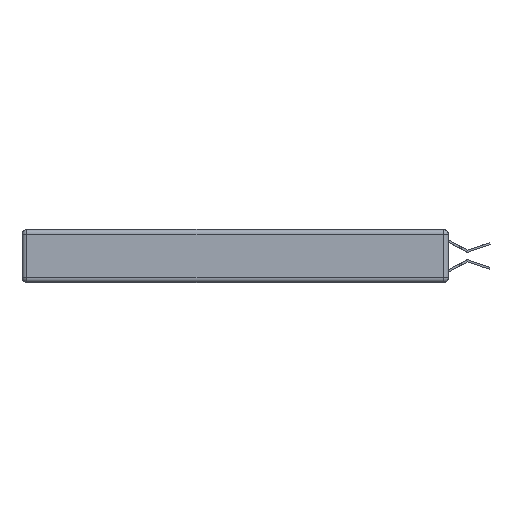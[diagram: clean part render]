
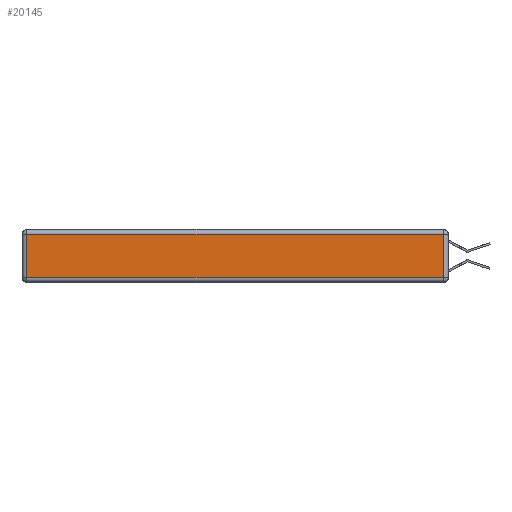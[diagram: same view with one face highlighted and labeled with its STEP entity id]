
A CAD part, left-side view. The second image highlights one B-rep face of the part: STEP entity #20145.
In plain terms, the highlighted planar face has unit normal (-1, 0, 0).
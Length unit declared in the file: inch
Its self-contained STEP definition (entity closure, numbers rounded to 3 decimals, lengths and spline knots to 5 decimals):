
#944 = DIRECTION ( 'NONE',  ( 0., 0., 1. ) ) ;
#1008 = ORIENTED_EDGE ( 'NONE', *, *, #22902, .T. ) ;
#3043 = CARTESIAN_POINT ( 'NONE',  ( 0., 0.03, -0.343 ) ) ;
#3604 = EDGE_LOOP ( 'NONE', ( #24940, #20591, #23111, #1008 ) ) ;
#4752 = EDGE_CURVE ( 'NONE', #14239, #12407, #6963, .T. ) ;
#5541 = LINE ( 'NONE', #11341, #27561 ) ;
#5569 = VECTOR ( 'NONE', #24279, 39.37008 ) ;
#5572 = DIRECTION ( 'NONE',  ( 0., -1., 0. ) ) ;
#6963 = LINE ( 'NONE', #3043, #24963 ) ;
#9137 = CARTESIAN_POINT ( 'NONE',  ( 0., 2.72, -0.313 ) ) ;
#10764 = EDGE_CURVE ( 'NONE', #12407, #19126, #21572, .T. ) ;
#11341 = CARTESIAN_POINT ( 'NONE',  ( 0., 2.72, -0.343 ) ) ;
#11521 = DIRECTION ( 'NONE',  ( 0., 0., -1. ) ) ;
#11660 = PLANE ( 'NONE',  #12733 ) ;
#12248 = DIRECTION ( 'NONE',  ( 0., 0., 1. ) ) ;
#12407 = VERTEX_POINT ( 'NONE', #17963 ) ;
#12733 = AXIS2_PLACEMENT_3D ( 'NONE', #19954, #22110, #944 ) ;
#14239 = VERTEX_POINT ( 'NONE', #20030 ) ;
#15270 = VERTEX_POINT ( 'NONE', #9137 ) ;
#17172 = LINE ( 'NONE', #18204, #23538 ) ;
#17803 = CARTESIAN_POINT ( 'NONE',  ( 0., 2.75, -0.03 ) ) ;
#17963 = CARTESIAN_POINT ( 'NONE',  ( 0., 0.03, -0.03 ) ) ;
#18204 = CARTESIAN_POINT ( 'NONE',  ( 0., 0., -0.313 ) ) ;
#18760 = CARTESIAN_POINT ( 'NONE',  ( 0., 2.72, -0.03 ) ) ;
#19126 = VERTEX_POINT ( 'NONE', #18760 ) ;
#19954 = CARTESIAN_POINT ( 'NONE',  ( 0., 0., -0.343 ) ) ;
#20030 = CARTESIAN_POINT ( 'NONE',  ( 0., 0.03, -0.313 ) ) ;
#20145 = ADVANCED_FACE ( 'NONE', ( #25808 ), #11660, .T. ) ;
#20591 = ORIENTED_EDGE ( 'NONE', *, *, #4752, .T. ) ;
#21572 = LINE ( 'NONE', #17803, #5569 ) ;
#22110 = DIRECTION ( 'NONE',  ( -1., 0., 0. ) ) ;
#22902 = EDGE_CURVE ( 'NONE', #19126, #15270, #5541, .T. ) ;
#23080 = EDGE_CURVE ( 'NONE', #15270, #14239, #17172, .T. ) ;
#23111 = ORIENTED_EDGE ( 'NONE', *, *, #10764, .T. ) ;
#23538 = VECTOR ( 'NONE', #5572, 39.37008 ) ;
#24279 = DIRECTION ( 'NONE',  ( 0., 1., 0. ) ) ;
#24940 = ORIENTED_EDGE ( 'NONE', *, *, #23080, .T. ) ;
#24963 = VECTOR ( 'NONE', #12248, 39.37008 ) ;
#25808 = FACE_OUTER_BOUND ( 'NONE', #3604, .T. ) ;
#27561 = VECTOR ( 'NONE', #11521, 39.37008 ) ;
